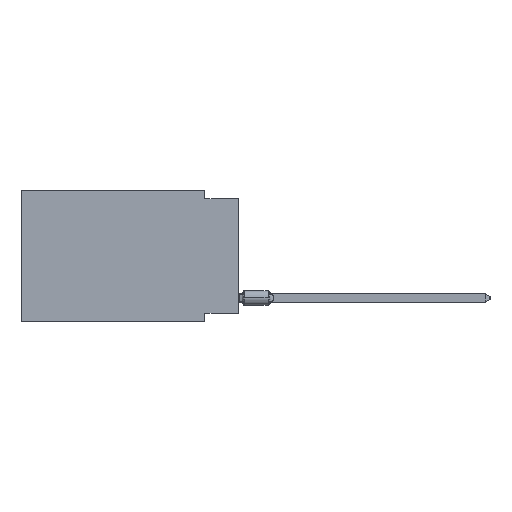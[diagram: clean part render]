
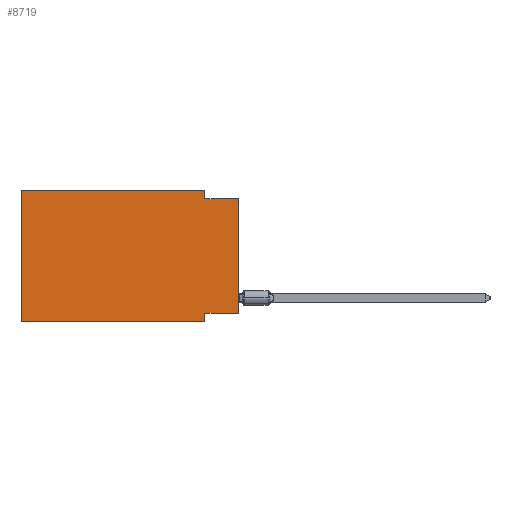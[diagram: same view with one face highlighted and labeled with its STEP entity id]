
A CAD part, left-side view. The second image highlights one B-rep face of the part: STEP entity #8719.
In plain terms, the highlighted planar face has unit normal (-1, 0, 0).
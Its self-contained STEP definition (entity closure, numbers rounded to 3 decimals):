
#355 = DIRECTION ( 'NONE',  ( 1., 0., 0. ) ) ;
#1281 = VERTEX_POINT ( 'NONE', #25305 ) ;
#1785 = ORIENTED_EDGE ( 'NONE', *, *, #34398, .F. ) ;
#1906 = ORIENTED_EDGE ( 'NONE', *, *, #51847, .F. ) ;
#1956 = CARTESIAN_POINT ( 'NONE',  ( 0., 0., -9.271 ) ) ;
#3341 = VECTOR ( 'NONE', #59758, 1000. ) ;
#3355 = CARTESIAN_POINT ( 'NONE',  ( 0., 16.383, -9.906 ) ) ;
#4610 = CARTESIAN_POINT ( 'NONE',  ( 0., 2.54, -9.906 ) ) ;
#5411 = LINE ( 'NONE', #4610, #29777 ) ;
#6968 = EDGE_CURVE ( 'NONE', #33596, #62488, #11108, .T. ) ;
#7251 = DIRECTION ( 'NONE',  ( 0., 1., 0. ) ) ;
#7301 = VERTEX_POINT ( 'NONE', #3355 ) ;
#8719 = ADVANCED_FACE ( 'NONE', ( #29886 ), #31073, .F. ) ;
#8922 = ORIENTED_EDGE ( 'NONE', *, *, #20451, .F. ) ;
#9182 = CARTESIAN_POINT ( 'NONE',  ( 0., 16.383, 0. ) ) ;
#10233 = EDGE_LOOP ( 'NONE', ( #71968, #1785, #75856, #8922, #1906, #46754, #65235, #71860 ) ) ;
#11108 = LINE ( 'NONE', #35758, #37300 ) ;
#13654 = LINE ( 'NONE', #74663, #44714 ) ;
#16225 = CARTESIAN_POINT ( 'NONE',  ( 0., 2.54, 0. ) ) ;
#16341 = LINE ( 'NONE', #77340, #55183 ) ;
#16445 = LINE ( 'NONE', #9182, #73657 ) ;
#16655 = AXIS2_PLACEMENT_3D ( 'NONE', #37520, #355, #54915 ) ;
#16815 = VECTOR ( 'NONE', #7251, 1000. ) ;
#18748 = DIRECTION ( 'NONE',  ( 0., -1., 0. ) ) ;
#19092 = EDGE_CURVE ( 'NONE', #48348, #1281, #27031, .T. ) ;
#20451 = EDGE_CURVE ( 'NONE', #26668, #33596, #16445, .T. ) ;
#21815 = CARTESIAN_POINT ( 'NONE',  ( 0., 0., 0. ) ) ;
#22414 = DIRECTION ( 'NONE',  ( 0., 0., -1. ) ) ;
#24812 = LINE ( 'NONE', #74086, #55379 ) ;
#25305 = CARTESIAN_POINT ( 'NONE',  ( 0., 2.54, -9.271 ) ) ;
#26668 = VERTEX_POINT ( 'NONE', #29559 ) ;
#27031 = LINE ( 'NONE', #1956, #16815 ) ;
#27621 = VERTEX_POINT ( 'NONE', #77640 ) ;
#28663 = LINE ( 'NONE', #21815, #3341 ) ;
#29559 = CARTESIAN_POINT ( 'NONE',  ( 0., 16.383, 0. ) ) ;
#29777 = VECTOR ( 'NONE', #22414, 1000. ) ;
#29886 = FACE_OUTER_BOUND ( 'NONE', #10233, .T. ) ;
#30807 = EDGE_CURVE ( 'NONE', #48348, #77880, #28663, .T. ) ;
#31073 = PLANE ( 'NONE',  #16655 ) ;
#33596 = VERTEX_POINT ( 'NONE', #16225 ) ;
#34398 = EDGE_CURVE ( 'NONE', #62488, #77880, #16341, .T. ) ;
#35010 = DIRECTION ( 'NONE',  ( 0., -1., 0. ) ) ;
#35758 = CARTESIAN_POINT ( 'NONE',  ( 0., 2.54, 0. ) ) ;
#37300 = VECTOR ( 'NONE', #77383, 1000. ) ;
#37520 = CARTESIAN_POINT ( 'NONE',  ( 0., 16.383, 0. ) ) ;
#38225 = CARTESIAN_POINT ( 'NONE',  ( 0., 2.54, -0.635 ) ) ;
#44714 = VECTOR ( 'NONE', #79535, 1000. ) ;
#46754 = ORIENTED_EDGE ( 'NONE', *, *, #72993, .T. ) ;
#47511 = CARTESIAN_POINT ( 'NONE',  ( 0., 0., -0.635 ) ) ;
#48348 = VERTEX_POINT ( 'NONE', #72245 ) ;
#51847 = EDGE_CURVE ( 'NONE', #7301, #26668, #13654, .T. ) ;
#53090 = DIRECTION ( 'NONE',  ( 0., -1., 0. ) ) ;
#54915 = DIRECTION ( 'NONE',  ( 0., 0., -1. ) ) ;
#55183 = VECTOR ( 'NONE', #53090, 1000. ) ;
#55379 = VECTOR ( 'NONE', #18748, 1000. ) ;
#59758 = DIRECTION ( 'NONE',  ( 0., 0., 1. ) ) ;
#62488 = VERTEX_POINT ( 'NONE', #38225 ) ;
#65235 = ORIENTED_EDGE ( 'NONE', *, *, #74289, .F. ) ;
#71860 = ORIENTED_EDGE ( 'NONE', *, *, #19092, .F. ) ;
#71968 = ORIENTED_EDGE ( 'NONE', *, *, #30807, .T. ) ;
#72245 = CARTESIAN_POINT ( 'NONE',  ( 0., 0., -9.271 ) ) ;
#72993 = EDGE_CURVE ( 'NONE', #7301, #27621, #24812, .T. ) ;
#73657 = VECTOR ( 'NONE', #35010, 1000. ) ;
#74086 = CARTESIAN_POINT ( 'NONE',  ( 0., 16.383, -9.906 ) ) ;
#74289 = EDGE_CURVE ( 'NONE', #1281, #27621, #5411, .T. ) ;
#74663 = CARTESIAN_POINT ( 'NONE',  ( 0., 16.383, 0. ) ) ;
#75856 = ORIENTED_EDGE ( 'NONE', *, *, #6968, .F. ) ;
#77340 = CARTESIAN_POINT ( 'NONE',  ( 0., 0., -0.635 ) ) ;
#77383 = DIRECTION ( 'NONE',  ( 0., 0., -1. ) ) ;
#77640 = CARTESIAN_POINT ( 'NONE',  ( 0., 2.54, -9.906 ) ) ;
#77880 = VERTEX_POINT ( 'NONE', #47511 ) ;
#79535 = DIRECTION ( 'NONE',  ( 0., 0., 1. ) ) ;
